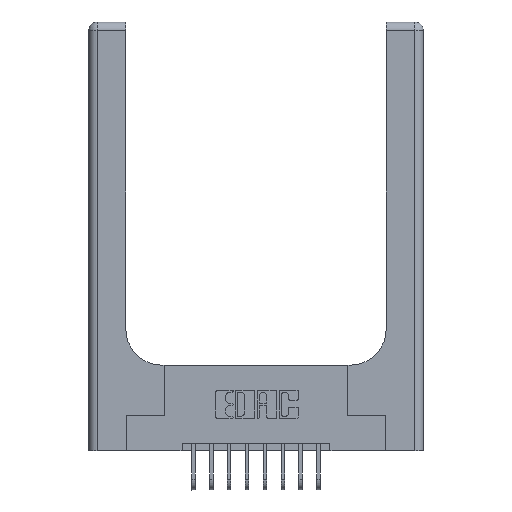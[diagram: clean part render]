
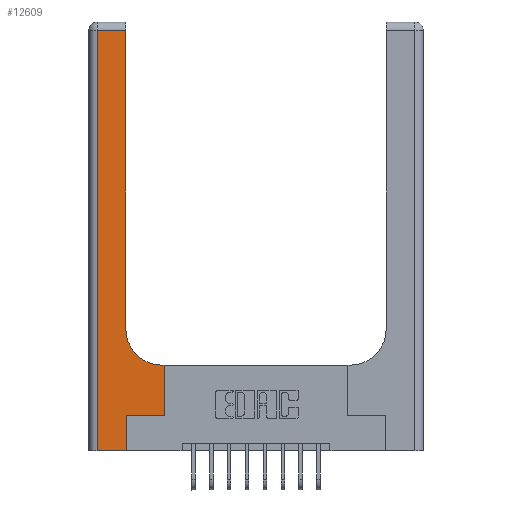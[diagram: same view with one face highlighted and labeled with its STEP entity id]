
A CAD part, top view. The second image highlights one B-rep face of the part: STEP entity #12609.
In plain terms, the highlighted planar face has unit normal (0, 0, 1).
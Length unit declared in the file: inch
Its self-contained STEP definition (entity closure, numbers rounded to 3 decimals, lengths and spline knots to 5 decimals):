
#276 = ORIENTED_EDGE ( 'NONE', *, *, #6749, .T. ) ;
#702 = VECTOR ( 'NONE', #16416, 39.37008 ) ;
#797 = VERTEX_POINT ( 'NONE', #1761 ) ;
#893 = CARTESIAN_POINT ( 'NONE',  ( 0.06, 0., 0.37 ) ) ;
#1412 = ORIENTED_EDGE ( 'NONE', *, *, #8485, .T. ) ;
#1439 = EDGE_CURVE ( 'NONE', #8044, #9912, #4906, .T. ) ;
#1533 = DIRECTION ( 'NONE',  ( 0., 0., -1. ) ) ;
#1656 = LINE ( 'NONE', #14916, #3299 ) ;
#1761 = CARTESIAN_POINT ( 'NONE',  ( 0.528, 0.25, 0.37 ) ) ;
#1848 = ORIENTED_EDGE ( 'NONE', *, *, #16384, .T. ) ;
#2052 = DIRECTION ( 'NONE',  ( 0., 1., 0. ) ) ;
#2164 = EDGE_CURVE ( 'NONE', #9912, #8582, #1656, .T. ) ;
#2342 = CARTESIAN_POINT ( 'NONE',  ( 0.528, 0.6, 0.37 ) ) ;
#2538 = CARTESIAN_POINT ( 'NONE',  ( 0., 2.94, 0.37 ) ) ;
#2757 = DIRECTION ( 'NONE',  ( 1., 0., 0. ) ) ;
#3247 = EDGE_CURVE ( 'NONE', #14143, #7781, #6531, .T. ) ;
#3299 = VECTOR ( 'NONE', #10642, 39.37008 ) ;
#3304 = DIRECTION ( 'NONE',  ( -1., 0., 0. ) ) ;
#3466 = CARTESIAN_POINT ( 'NONE',  ( 0., 3., 0.37 ) ) ;
#3815 = CARTESIAN_POINT ( 'NONE',  ( 0.06, 3., 0.37 ) ) ;
#4178 = EDGE_CURVE ( 'NONE', #797, #8168, #16082, .T. ) ;
#4892 = CARTESIAN_POINT ( 'NONE',  ( 0.528, 0.25, 0.37 ) ) ;
#4906 = LINE ( 'NONE', #14776, #14227 ) ;
#4908 = LINE ( 'NONE', #9613, #14028 ) ;
#5059 = EDGE_CURVE ( 'NONE', #8168, #14143, #9233, .T. ) ;
#5120 = LINE ( 'NONE', #2538, #9947 ) ;
#5185 = ORIENTED_EDGE ( 'NONE', *, *, #3247, .T. ) ;
#5734 = ORIENTED_EDGE ( 'NONE', *, *, #4178, .T. ) ;
#6040 = CARTESIAN_POINT ( 'NONE',  ( 0.265, 0.25, 0.37 ) ) ;
#6531 = CIRCLE ( 'NONE', #9853, 0.25 ) ;
#6749 = EDGE_CURVE ( 'NONE', #11074, #11043, #5120, .T. ) ;
#7781 = VERTEX_POINT ( 'NONE', #8075 ) ;
#7870 = ORIENTED_EDGE ( 'NONE', *, *, #15734, .T. ) ;
#7874 = AXIS2_PLACEMENT_3D ( 'NONE', #3466, #8572, #3304 ) ;
#7937 = VECTOR ( 'NONE', #14298, 39.37008 ) ;
#8044 = VERTEX_POINT ( 'NONE', #893 ) ;
#8075 = CARTESIAN_POINT ( 'NONE',  ( 0.26, 0.85, 0.37 ) ) ;
#8168 = VERTEX_POINT ( 'NONE', #2342 ) ;
#8485 = EDGE_CURVE ( 'NONE', #8582, #797, #4908, .T. ) ;
#8572 = DIRECTION ( 'NONE',  ( 0., 0., -1. ) ) ;
#8582 = VERTEX_POINT ( 'NONE', #6040 ) ;
#9083 = ORIENTED_EDGE ( 'NONE', *, *, #1439, .T. ) ;
#9233 = LINE ( 'NONE', #15235, #702 ) ;
#9613 = CARTESIAN_POINT ( 'NONE',  ( 0.265, 0.25, 0.37 ) ) ;
#9853 = AXIS2_PLACEMENT_3D ( 'NONE', #15832, #1533, #2757 ) ;
#9912 = VERTEX_POINT ( 'NONE', #15788 ) ;
#9914 = PLANE ( 'NONE',  #7874 ) ;
#9947 = VECTOR ( 'NONE', #11597, 39.37008 ) ;
#10233 = DIRECTION ( 'NONE',  ( 0., 1., 0. ) ) ;
#10642 = DIRECTION ( 'NONE',  ( 0., 1., 0. ) ) ;
#11043 = VERTEX_POINT ( 'NONE', #11828 ) ;
#11074 = VERTEX_POINT ( 'NONE', #14602 ) ;
#11416 = ORIENTED_EDGE ( 'NONE', *, *, #2164, .T. ) ;
#11421 = VECTOR ( 'NONE', #10233, 39.37008 ) ;
#11597 = DIRECTION ( 'NONE',  ( -1., 0., 0. ) ) ;
#11704 = VECTOR ( 'NONE', #2052, 39.37008 ) ;
#11828 = CARTESIAN_POINT ( 'NONE',  ( 0.06, 2.94, 0.37 ) ) ;
#12104 = EDGE_LOOP ( 'NONE', ( #7870, #276, #1848, #9083, #11416, #1412, #5734, #15442, #5185 ) ) ;
#12184 = CARTESIAN_POINT ( 'NONE',  ( 0.26, 3., 0.37 ) ) ;
#12609 = ADVANCED_FACE ( 'NONE', ( #15619 ), #9914, .F. ) ;
#12714 = LINE ( 'NONE', #12184, #11704 ) ;
#13596 = DIRECTION ( 'NONE',  ( 1., 0., 0. ) ) ;
#13662 = LINE ( 'NONE', #3815, #7937 ) ;
#14028 = VECTOR ( 'NONE', #13596, 39.37008 ) ;
#14143 = VERTEX_POINT ( 'NONE', #16278 ) ;
#14227 = VECTOR ( 'NONE', #14508, 39.37008 ) ;
#14298 = DIRECTION ( 'NONE',  ( 0., -1., 0. ) ) ;
#14508 = DIRECTION ( 'NONE',  ( 1., 0., 0. ) ) ;
#14602 = CARTESIAN_POINT ( 'NONE',  ( 0.26, 2.94, 0.37 ) ) ;
#14776 = CARTESIAN_POINT ( 'NONE',  ( 0., 0., 0.37 ) ) ;
#14916 = CARTESIAN_POINT ( 'NONE',  ( 0.265, 0., 0.37 ) ) ;
#15235 = CARTESIAN_POINT ( 'NONE',  ( 0.26, 0.6, 0.37 ) ) ;
#15442 = ORIENTED_EDGE ( 'NONE', *, *, #5059, .T. ) ;
#15619 = FACE_OUTER_BOUND ( 'NONE', #12104, .T. ) ;
#15734 = EDGE_CURVE ( 'NONE', #7781, #11074, #12714, .T. ) ;
#15788 = CARTESIAN_POINT ( 'NONE',  ( 0.265, 0., 0.37 ) ) ;
#15832 = CARTESIAN_POINT ( 'NONE',  ( 0.51, 0.85, 0.37 ) ) ;
#16082 = LINE ( 'NONE', #4892, #11421 ) ;
#16278 = CARTESIAN_POINT ( 'NONE',  ( 0.51, 0.6, 0.37 ) ) ;
#16384 = EDGE_CURVE ( 'NONE', #11043, #8044, #13662, .T. ) ;
#16416 = DIRECTION ( 'NONE',  ( -1., 0., 0. ) ) ;
